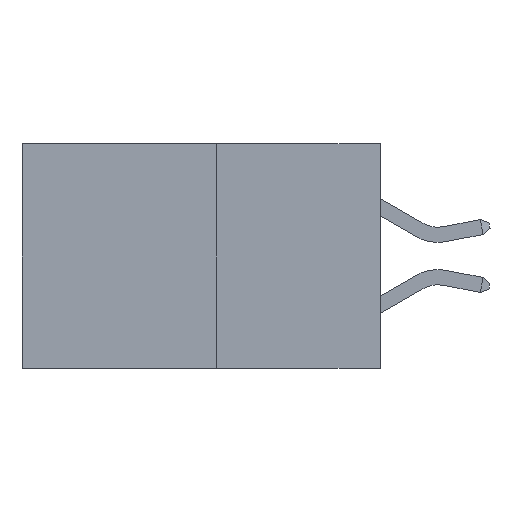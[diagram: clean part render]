
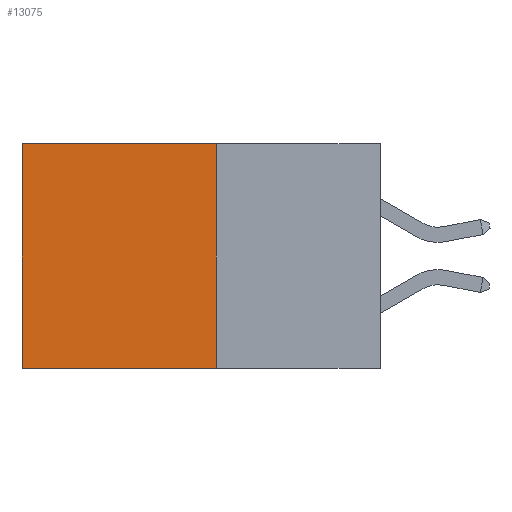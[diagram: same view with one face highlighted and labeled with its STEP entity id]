
A CAD part, left-side view. The second image highlights one B-rep face of the part: STEP entity #13075.
In plain terms, the highlighted planar face has unit normal (-1, 0, 0).
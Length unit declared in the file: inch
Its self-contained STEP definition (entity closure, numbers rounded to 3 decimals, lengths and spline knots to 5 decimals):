
#1214 = CARTESIAN_POINT ( 'NONE',  ( 0.277, 0.27, -0.37 ) ) ;
#3946 = ORIENTED_EDGE ( 'NONE', *, *, #17905, .T. ) ;
#6944 = CARTESIAN_POINT ( 'NONE',  ( 0.277, 0.27, 0. ) ) ;
#7639 = VECTOR ( 'NONE', #27749, 39.37008 ) ;
#8198 = VERTEX_POINT ( 'NONE', #34877 ) ;
#8719 = CARTESIAN_POINT ( 'NONE',  ( 0.277, 0.59, -0.37 ) ) ;
#9691 = CARTESIAN_POINT ( 'NONE',  ( 0.277, 0.27, 0. ) ) ;
#10620 = LINE ( 'NONE', #24507, #24314 ) ;
#11398 = CARTESIAN_POINT ( 'NONE',  ( 0.277, 0.27, -0.37 ) ) ;
#11511 = PLANE ( 'NONE',  #23581 ) ;
#12663 = VERTEX_POINT ( 'NONE', #1214 ) ;
#13075 = ADVANCED_FACE ( 'NONE', ( #31876 ), #11511, .F. ) ;
#14003 = EDGE_LOOP ( 'NONE', ( #3946, #16219, #19172, #15951 ) ) ;
#14246 = DIRECTION ( 'NONE',  ( 1., 0., 0. ) ) ;
#15951 = ORIENTED_EDGE ( 'NONE', *, *, #21411, .T. ) ;
#16219 = ORIENTED_EDGE ( 'NONE', *, *, #23158, .F. ) ;
#17905 = EDGE_CURVE ( 'NONE', #8198, #21222, #20797, .T. ) ;
#18362 = VERTEX_POINT ( 'NONE', #6944 ) ;
#19172 = ORIENTED_EDGE ( 'NONE', *, *, #23733, .F. ) ;
#20667 = DIRECTION ( 'NONE',  ( 0., 1., 0. ) ) ;
#20797 = LINE ( 'NONE', #8719, #34412 ) ;
#21222 = VERTEX_POINT ( 'NONE', #27987 ) ;
#21411 = EDGE_CURVE ( 'NONE', #18362, #8198, #29514, .T. ) ;
#23158 = EDGE_CURVE ( 'NONE', #12663, #21222, #29467, .T. ) ;
#23581 = AXIS2_PLACEMENT_3D ( 'NONE', #11398, #14246, #33321 ) ;
#23733 = EDGE_CURVE ( 'NONE', #18362, #12663, #10620, .T. ) ;
#24314 = VECTOR ( 'NONE', #27229, 39.37008 ) ;
#24507 = CARTESIAN_POINT ( 'NONE',  ( 0.277, 0.27, -0.37 ) ) ;
#25009 = CARTESIAN_POINT ( 'NONE',  ( 0.277, 0.27, -0.37 ) ) ;
#27229 = DIRECTION ( 'NONE',  ( 0., 0., -1. ) ) ;
#27749 = DIRECTION ( 'NONE',  ( 0., 1., 0. ) ) ;
#27987 = CARTESIAN_POINT ( 'NONE',  ( 0.277, 0.59, -0.37 ) ) ;
#28682 = VECTOR ( 'NONE', #20667, 39.37008 ) ;
#29467 = LINE ( 'NONE', #25009, #7639 ) ;
#29514 = LINE ( 'NONE', #9691, #28682 ) ;
#30560 = DIRECTION ( 'NONE',  ( 0., 0., -1. ) ) ;
#31876 = FACE_OUTER_BOUND ( 'NONE', #14003, .T. ) ;
#33321 = DIRECTION ( 'NONE',  ( 0., 0., -1. ) ) ;
#34412 = VECTOR ( 'NONE', #30560, 39.37008 ) ;
#34877 = CARTESIAN_POINT ( 'NONE',  ( 0.277, 0.59, 0. ) ) ;
